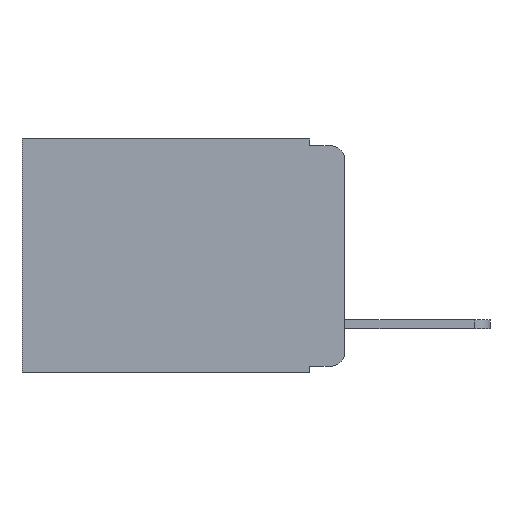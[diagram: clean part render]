
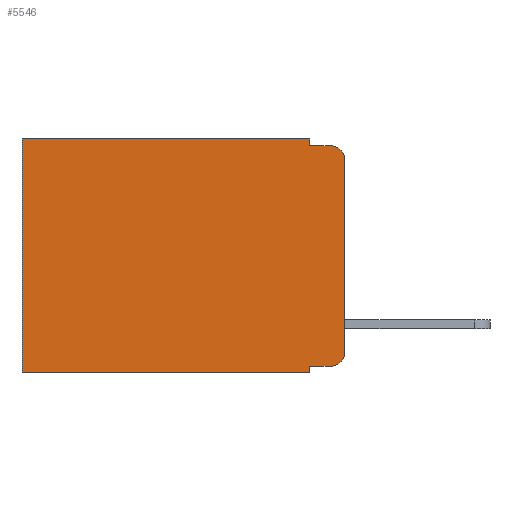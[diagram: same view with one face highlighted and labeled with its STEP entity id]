
A CAD part, left-side view. The second image highlights one B-rep face of the part: STEP entity #5546.
In plain terms, the highlighted planar face has unit normal (-1, 0, 0).
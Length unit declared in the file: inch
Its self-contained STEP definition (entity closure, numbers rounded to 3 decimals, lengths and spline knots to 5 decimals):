
#136 = CARTESIAN_POINT ( 'NONE',  ( 0.298, 0.051, -0.333 ) ) ;
#190 = DIRECTION ( 'NONE',  ( 0., -1., 0. ) ) ;
#230 = CARTESIAN_POINT ( 'NONE',  ( 0.298, 0.051, -0.01 ) ) ;
#276 = VECTOR ( 'NONE', #8907, 39.37008 ) ;
#445 = EDGE_CURVE ( 'NONE', #13990, #9091, #10841, .T. ) ;
#485 = DIRECTION ( 'NONE',  ( 0., 0., -1. ) ) ;
#591 = CARTESIAN_POINT ( 'NONE',  ( 0.298, 0.051, 0. ) ) ;
#901 = CARTESIAN_POINT ( 'NONE',  ( 0.298, 0., -0.03 ) ) ;
#1234 = DIRECTION ( 'NONE',  ( -1., 0., 0. ) ) ;
#1254 = VERTEX_POINT ( 'NONE', #1916 ) ;
#1521 = VERTEX_POINT ( 'NONE', #2717 ) ;
#1759 = PLANE ( 'NONE',  #9747 ) ;
#1766 = ORIENTED_EDGE ( 'NONE', *, *, #4304, .F. ) ;
#1916 = CARTESIAN_POINT ( 'NONE',  ( 0.298, 0.051, -0.333 ) ) ;
#2183 = CARTESIAN_POINT ( 'NONE',  ( 0.298, 0., 0. ) ) ;
#2303 = CARTESIAN_POINT ( 'NONE',  ( 0.298, 0.051, -0.343 ) ) ;
#2582 = CARTESIAN_POINT ( 'NONE',  ( 0.298, 0.02, -0.01 ) ) ;
#2596 = DIRECTION ( 'NONE',  ( 1., 0., 0. ) ) ;
#2717 = CARTESIAN_POINT ( 'NONE',  ( 0.298, 0.473, 0. ) ) ;
#2806 = EDGE_CURVE ( 'NONE', #1521, #11051, #4090, .T. ) ;
#2890 = LINE ( 'NONE', #136, #11297 ) ;
#3589 = EDGE_CURVE ( 'NONE', #5029, #13990, #5847, .T. ) ;
#3593 = AXIS2_PLACEMENT_3D ( 'NONE', #6233, #13638, #7319 ) ;
#3673 = EDGE_CURVE ( 'NONE', #5029, #1521, #7736, .T. ) ;
#3897 = ORIENTED_EDGE ( 'NONE', *, *, #3589, .F. ) ;
#4012 = VECTOR ( 'NONE', #6704, 39.37008 ) ;
#4090 = LINE ( 'NONE', #6775, #9639 ) ;
#4248 = ORIENTED_EDGE ( 'NONE', *, *, #3673, .T. ) ;
#4304 = EDGE_CURVE ( 'NONE', #1254, #8408, #9883, .T. ) ;
#4526 = CARTESIAN_POINT ( 'NONE',  ( 0.298, 0.051, 0. ) ) ;
#5029 = VERTEX_POINT ( 'NONE', #591 ) ;
#5119 = ORIENTED_EDGE ( 'NONE', *, *, #7303, .T. ) ;
#5129 = CARTESIAN_POINT ( 'NONE',  ( 0.298, 0.473, -0.343 ) ) ;
#5259 = CARTESIAN_POINT ( 'NONE',  ( 0.298, 0., 0. ) ) ;
#5339 = CARTESIAN_POINT ( 'NONE',  ( 0.298, 0., 0. ) ) ;
#5530 = DIRECTION ( 'NONE',  ( 0., 1., 0. ) ) ;
#5546 = ADVANCED_FACE ( 'NONE', ( #5746 ), #1759, .F. ) ;
#5746 = FACE_OUTER_BOUND ( 'NONE', #6851, .T. ) ;
#5847 = LINE ( 'NONE', #4526, #11252 ) ;
#5968 = CARTESIAN_POINT ( 'NONE',  ( 0.298, 0., -0.313 ) ) ;
#5994 = VERTEX_POINT ( 'NONE', #901 ) ;
#5999 = AXIS2_PLACEMENT_3D ( 'NONE', #7971, #1234, #9087 ) ;
#6113 = DIRECTION ( 'NONE',  ( 0., 1., 0. ) ) ;
#6233 = CARTESIAN_POINT ( 'NONE',  ( 0.298, 0.02, -0.313 ) ) ;
#6704 = DIRECTION ( 'NONE',  ( 0., 0., -1. ) ) ;
#6746 = DIRECTION ( 'NONE',  ( 0., 0., -1. ) ) ;
#6775 = CARTESIAN_POINT ( 'NONE',  ( 0.298, 0.473, 0. ) ) ;
#6851 = EDGE_LOOP ( 'NONE', ( #10609, #10946, #12248, #3897, #4248, #10113, #13005, #1766, #5119, #10928 ) ) ;
#7192 = CARTESIAN_POINT ( 'NONE',  ( 0.298, 0., -0.343 ) ) ;
#7303 = EDGE_CURVE ( 'NONE', #1254, #8511, #2890, .T. ) ;
#7319 = DIRECTION ( 'NONE',  ( 0., 0., -1. ) ) ;
#7543 = CIRCLE ( 'NONE', #5999, 0.02 ) ;
#7736 = LINE ( 'NONE', #5259, #12701 ) ;
#7971 = CARTESIAN_POINT ( 'NONE',  ( 0.298, 0.02, -0.03 ) ) ;
#8056 = EDGE_CURVE ( 'NONE', #8511, #9777, #10466, .T. ) ;
#8408 = VERTEX_POINT ( 'NONE', #2303 ) ;
#8511 = VERTEX_POINT ( 'NONE', #10487 ) ;
#8902 = DIRECTION ( 'NONE',  ( 0., -1., 0. ) ) ;
#8907 = DIRECTION ( 'NONE',  ( 0., 0., -1. ) ) ;
#9087 = DIRECTION ( 'NONE',  ( 0., 0., -1. ) ) ;
#9091 = VERTEX_POINT ( 'NONE', #2582 ) ;
#9639 = VECTOR ( 'NONE', #6746, 39.37008 ) ;
#9643 = LINE ( 'NONE', #2183, #276 ) ;
#9747 = AXIS2_PLACEMENT_3D ( 'NONE', #5339, #2596, #485 ) ;
#9777 = VERTEX_POINT ( 'NONE', #5968 ) ;
#9883 = LINE ( 'NONE', #9919, #4012 ) ;
#9919 = CARTESIAN_POINT ( 'NONE',  ( 0.298, 0.051, 0. ) ) ;
#10113 = ORIENTED_EDGE ( 'NONE', *, *, #2806, .T. ) ;
#10466 = CIRCLE ( 'NONE', #3593, 0.02 ) ;
#10479 = VECTOR ( 'NONE', #6113, 39.37008 ) ;
#10487 = CARTESIAN_POINT ( 'NONE',  ( 0.298, 0.02, -0.333 ) ) ;
#10514 = VECTOR ( 'NONE', #8902, 39.37008 ) ;
#10609 = ORIENTED_EDGE ( 'NONE', *, *, #11880, .F. ) ;
#10808 = LINE ( 'NONE', #7192, #10479 ) ;
#10841 = LINE ( 'NONE', #230, #10514 ) ;
#10928 = ORIENTED_EDGE ( 'NONE', *, *, #8056, .T. ) ;
#10946 = ORIENTED_EDGE ( 'NONE', *, *, #13243, .T. ) ;
#11051 = VERTEX_POINT ( 'NONE', #5129 ) ;
#11252 = VECTOR ( 'NONE', #11310, 39.37008 ) ;
#11297 = VECTOR ( 'NONE', #190, 39.37008 ) ;
#11310 = DIRECTION ( 'NONE',  ( 0., 0., -1. ) ) ;
#11433 = CARTESIAN_POINT ( 'NONE',  ( 0.298, 0.051, -0.01 ) ) ;
#11558 = EDGE_CURVE ( 'NONE', #8408, #11051, #10808, .T. ) ;
#11880 = EDGE_CURVE ( 'NONE', #5994, #9777, #9643, .T. ) ;
#12248 = ORIENTED_EDGE ( 'NONE', *, *, #445, .F. ) ;
#12701 = VECTOR ( 'NONE', #5530, 39.37008 ) ;
#13005 = ORIENTED_EDGE ( 'NONE', *, *, #11558, .F. ) ;
#13243 = EDGE_CURVE ( 'NONE', #5994, #9091, #7543, .T. ) ;
#13638 = DIRECTION ( 'NONE',  ( -1., 0., 0. ) ) ;
#13990 = VERTEX_POINT ( 'NONE', #11433 ) ;
